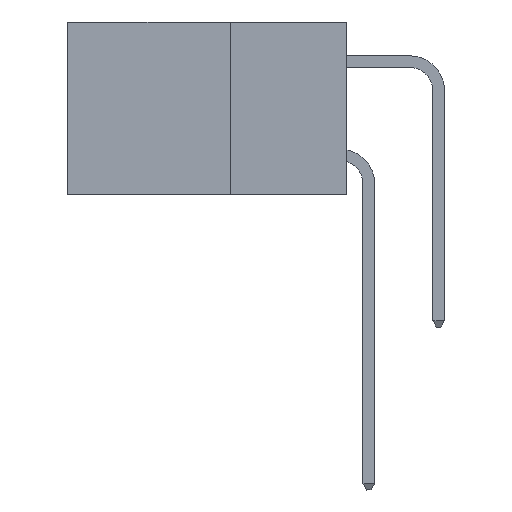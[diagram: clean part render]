
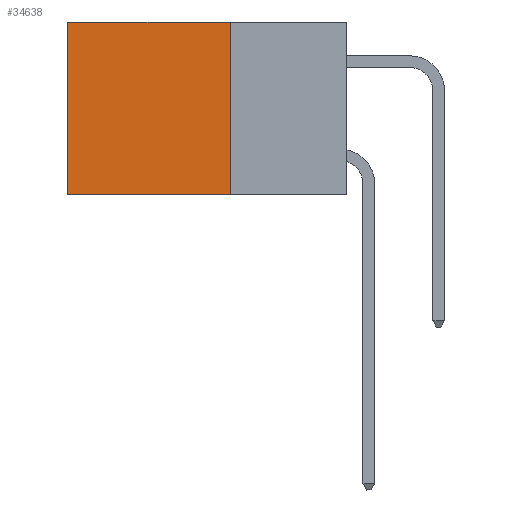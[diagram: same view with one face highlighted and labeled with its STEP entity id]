
A CAD part, left-side view. The second image highlights one B-rep face of the part: STEP entity #34638.
In plain terms, the highlighted planar face has unit normal (-1, 0, 0).
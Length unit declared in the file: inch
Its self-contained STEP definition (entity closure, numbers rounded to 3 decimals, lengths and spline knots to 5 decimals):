
#1463 = CARTESIAN_POINT ( 'NONE',  ( 0.2875, 0.6, 0. ) ) ;
#1998 = CARTESIAN_POINT ( 'NONE',  ( 0.2875, 0.6, 0. ) ) ;
#2442 = ORIENTED_EDGE ( 'NONE', *, *, #27614, .T. ) ;
#2491 = DIRECTION ( 'NONE',  ( 0., 0., -1. ) ) ;
#7621 = ORIENTED_EDGE ( 'NONE', *, *, #7783, .T. ) ;
#7783 = EDGE_CURVE ( 'NONE', #9563, #13695, #31208, .T. ) ;
#7911 = CARTESIAN_POINT ( 'NONE',  ( 0.2875, 0.25, -0.37 ) ) ;
#9281 = CARTESIAN_POINT ( 'NONE',  ( 0.2875, 0.25, 0. ) ) ;
#9563 = VERTEX_POINT ( 'NONE', #1463 ) ;
#10588 = CARTESIAN_POINT ( 'NONE',  ( 0.2875, 0.6, -0.37 ) ) ;
#12082 = DIRECTION ( 'NONE',  ( 0., 1., 0. ) ) ;
#12666 = VECTOR ( 'NONE', #26473, 39.37008 ) ;
#12796 = DIRECTION ( 'NONE',  ( 0., 0., -1. ) ) ;
#13695 = VERTEX_POINT ( 'NONE', #10588 ) ;
#15563 = ORIENTED_EDGE ( 'NONE', *, *, #23913, .F. ) ;
#18467 = AXIS2_PLACEMENT_3D ( 'NONE', #44119, #23482, #2491 ) ;
#18608 = FACE_OUTER_BOUND ( 'NONE', #21496, .T. ) ;
#18958 = CARTESIAN_POINT ( 'NONE',  ( 0.2875, 0.25, 0. ) ) ;
#19576 = ORIENTED_EDGE ( 'NONE', *, *, #32689, .F. ) ;
#21496 = EDGE_LOOP ( 'NONE', ( #7621, #15563, #19576, #2442 ) ) ;
#23482 = DIRECTION ( 'NONE',  ( 1., 0., 0. ) ) ;
#23913 = EDGE_CURVE ( 'NONE', #25762, #13695, #43425, .T. ) ;
#25468 = CARTESIAN_POINT ( 'NONE',  ( 0.2875, 0.25, -0.37 ) ) ;
#25762 = VERTEX_POINT ( 'NONE', #7911 ) ;
#26473 = DIRECTION ( 'NONE',  ( 0., 0., -1. ) ) ;
#27588 = VERTEX_POINT ( 'NONE', #18958 ) ;
#27614 = EDGE_CURVE ( 'NONE', #27588, #9563, #39899, .T. ) ;
#30324 = PLANE ( 'NONE',  #18467 ) ;
#31208 = LINE ( 'NONE', #1998, #12666 ) ;
#32596 = DIRECTION ( 'NONE',  ( 0., 1., 0. ) ) ;
#32689 = EDGE_CURVE ( 'NONE', #27588, #25762, #33956, .T. ) ;
#33956 = LINE ( 'NONE', #9281, #35030 ) ;
#34300 = VECTOR ( 'NONE', #32596, 39.37008 ) ;
#34638 = ADVANCED_FACE ( 'NONE', ( #18608 ), #30324, .F. ) ;
#35030 = VECTOR ( 'NONE', #12796, 39.37008 ) ;
#36414 = CARTESIAN_POINT ( 'NONE',  ( 0.2875, 0.25, 0. ) ) ;
#38794 = VECTOR ( 'NONE', #12082, 39.37008 ) ;
#39899 = LINE ( 'NONE', #36414, #38794 ) ;
#43425 = LINE ( 'NONE', #25468, #34300 ) ;
#44119 = CARTESIAN_POINT ( 'NONE',  ( 0.2875, 0.25, 0. ) ) ;
